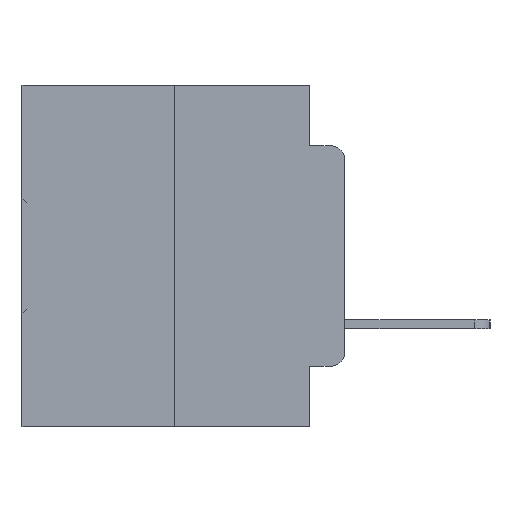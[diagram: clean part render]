
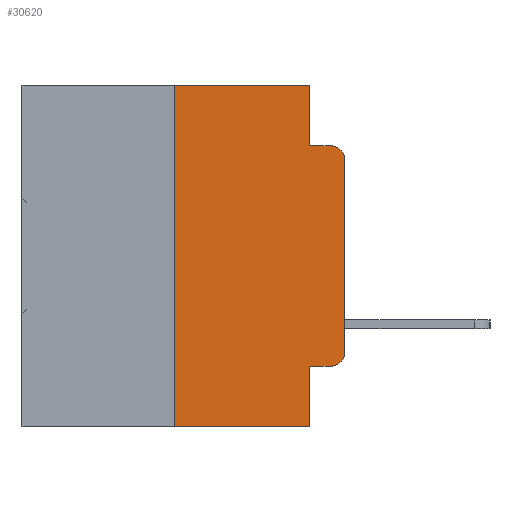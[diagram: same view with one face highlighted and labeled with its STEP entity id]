
A CAD part, left-side view. The second image highlights one B-rep face of the part: STEP entity #30620.
In plain terms, the highlighted planar face has unit normal (-1, 0, 0).
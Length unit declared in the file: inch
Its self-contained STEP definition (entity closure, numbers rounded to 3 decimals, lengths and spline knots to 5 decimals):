
#858 = EDGE_CURVE ( 'NONE', #8218, #5733, #8881, .T. ) ;
#883 = LINE ( 'NONE', #3838, #12982 ) ;
#1168 = EDGE_CURVE ( 'NONE', #4588, #17479, #20511, .T. ) ;
#2217 = DIRECTION ( 'NONE',  ( 0., 0., -1. ) ) ;
#2550 = DIRECTION ( 'NONE',  ( -1., 0., 0. ) ) ;
#2579 = ORIENTED_EDGE ( 'NONE', *, *, #3628, .T. ) ;
#2965 = LINE ( 'NONE', #25758, #28942 ) ;
#3628 = EDGE_CURVE ( 'NONE', #4588, #26644, #7631, .T. ) ;
#3838 = CARTESIAN_POINT ( 'NONE',  ( 0., 0.051, -0.0885 ) ) ;
#4324 = DIRECTION ( 'NONE',  ( 0., 0., 1. ) ) ;
#4588 = VERTEX_POINT ( 'NONE', #18211 ) ;
#5226 = EDGE_CURVE ( 'NONE', #5733, #17076, #21538, .T. ) ;
#5264 = EDGE_CURVE ( 'NONE', #19134, #17076, #883, .T. ) ;
#5346 = DIRECTION ( 'NONE',  ( 0., 0., 1. ) ) ;
#5366 = EDGE_CURVE ( 'NONE', #23782, #19134, #2965, .T. ) ;
#5705 = DIRECTION ( 'NONE',  ( -1., 0., 0. ) ) ;
#5733 = VERTEX_POINT ( 'NONE', #20081 ) ;
#5838 = VECTOR ( 'NONE', #27676, 39.37008 ) ;
#5846 = CARTESIAN_POINT ( 'NONE',  ( 0., 0.473, 0. ) ) ;
#5957 = LINE ( 'NONE', #25473, #25893 ) ;
#6396 = AXIS2_PLACEMENT_3D ( 'NONE', #17402, #5705, #10441 ) ;
#7501 = CARTESIAN_POINT ( 'NONE',  ( 0., 0.051, -0.4115 ) ) ;
#7631 = LINE ( 'NONE', #7501, #32658 ) ;
#7640 = VERTEX_POINT ( 'NONE', #32316 ) ;
#7984 = DIRECTION ( 'NONE',  ( 0., -1., 0. ) ) ;
#8181 = CARTESIAN_POINT ( 'NONE',  ( 0., 0.02, -0.4115 ) ) ;
#8218 = VERTEX_POINT ( 'NONE', #31843 ) ;
#8352 = PLANE ( 'NONE',  #21915 ) ;
#8881 = LINE ( 'NONE', #20272, #22927 ) ;
#9037 = EDGE_CURVE ( 'NONE', #7640, #10175, #15525, .T. ) ;
#9444 = ORIENTED_EDGE ( 'NONE', *, *, #21715, .T. ) ;
#10175 = VERTEX_POINT ( 'NONE', #11527 ) ;
#10441 = DIRECTION ( 'NONE',  ( 0., 0., -1. ) ) ;
#11527 = CARTESIAN_POINT ( 'NONE',  ( 0., 0.25, 0. ) ) ;
#12526 = LINE ( 'NONE', #17604, #5838 ) ;
#12982 = VECTOR ( 'NONE', #28740, 39.37008 ) ;
#13798 = ORIENTED_EDGE ( 'NONE', *, *, #9037, .F. ) ;
#15057 = CARTESIAN_POINT ( 'NONE',  ( 0., 0.051, 0. ) ) ;
#15525 = LINE ( 'NONE', #19328, #24042 ) ;
#15958 = CARTESIAN_POINT ( 'NONE',  ( 0., 0.051, -0.0885 ) ) ;
#17076 = VERTEX_POINT ( 'NONE', #27655 ) ;
#17402 = CARTESIAN_POINT ( 'NONE',  ( 0., 0.02, -0.1085 ) ) ;
#17479 = VERTEX_POINT ( 'NONE', #31328 ) ;
#17604 = CARTESIAN_POINT ( 'NONE',  ( 0., 0.473, -0.5 ) ) ;
#17721 = CARTESIAN_POINT ( 'NONE',  ( 0., 0.02, -0.3915 ) ) ;
#18211 = CARTESIAN_POINT ( 'NONE',  ( 0., 0.051, -0.4115 ) ) ;
#18778 = ORIENTED_EDGE ( 'NONE', *, *, #5366, .F. ) ;
#19088 = CIRCLE ( 'NONE', #28227, 0.02 ) ;
#19134 = VERTEX_POINT ( 'NONE', #15958 ) ;
#19328 = CARTESIAN_POINT ( 'NONE',  ( 0., 0.25, 0. ) ) ;
#19840 = FACE_OUTER_BOUND ( 'NONE', #25358, .T. ) ;
#20081 = CARTESIAN_POINT ( 'NONE',  ( 0., 0., -0.1085 ) ) ;
#20176 = DIRECTION ( 'NONE',  ( 0., 0., -1. ) ) ;
#20272 = CARTESIAN_POINT ( 'NONE',  ( 0., 0., 0. ) ) ;
#20511 = LINE ( 'NONE', #15057, #26450 ) ;
#20934 = CARTESIAN_POINT ( 'NONE',  ( 0., 0.051, 0. ) ) ;
#21538 = CIRCLE ( 'NONE', #6396, 0.02 ) ;
#21711 = EDGE_CURVE ( 'NONE', #7640, #17479, #12526, .T. ) ;
#21715 = EDGE_CURVE ( 'NONE', #26644, #8218, #19088, .T. ) ;
#21895 = ORIENTED_EDGE ( 'NONE', *, *, #1168, .F. ) ;
#21915 = AXIS2_PLACEMENT_3D ( 'NONE', #5846, #23184, #25831 ) ;
#22913 = DIRECTION ( 'NONE',  ( 0., 0., -1. ) ) ;
#22927 = VECTOR ( 'NONE', #5346, 39.37008 ) ;
#23184 = DIRECTION ( 'NONE',  ( 1., 0., 0. ) ) ;
#23782 = VERTEX_POINT ( 'NONE', #20934 ) ;
#23864 = ORIENTED_EDGE ( 'NONE', *, *, #5226, .T. ) ;
#24042 = VECTOR ( 'NONE', #4324, 39.37008 ) ;
#24340 = EDGE_CURVE ( 'NONE', #10175, #23782, #5957, .T. ) ;
#25358 = EDGE_LOOP ( 'NONE', ( #28180, #23864, #30517, #18778, #32089, #13798, #27041, #21895, #2579, #9444 ) ) ;
#25473 = CARTESIAN_POINT ( 'NONE',  ( 0., 0.473, 0. ) ) ;
#25758 = CARTESIAN_POINT ( 'NONE',  ( 0., 0.051, 0. ) ) ;
#25831 = DIRECTION ( 'NONE',  ( 0., 0., -1. ) ) ;
#25893 = VECTOR ( 'NONE', #7984, 39.37008 ) ;
#26450 = VECTOR ( 'NONE', #22913, 39.37008 ) ;
#26644 = VERTEX_POINT ( 'NONE', #8181 ) ;
#27041 = ORIENTED_EDGE ( 'NONE', *, *, #21711, .T. ) ;
#27655 = CARTESIAN_POINT ( 'NONE',  ( 0., 0.02, -0.0885 ) ) ;
#27676 = DIRECTION ( 'NONE',  ( 0., -1., 0. ) ) ;
#28180 = ORIENTED_EDGE ( 'NONE', *, *, #858, .T. ) ;
#28227 = AXIS2_PLACEMENT_3D ( 'NONE', #17721, #2550, #20176 ) ;
#28740 = DIRECTION ( 'NONE',  ( 0., -1., 0. ) ) ;
#28942 = VECTOR ( 'NONE', #2217, 39.37008 ) ;
#30517 = ORIENTED_EDGE ( 'NONE', *, *, #5264, .F. ) ;
#30598 = DIRECTION ( 'NONE',  ( 0., -1., 0. ) ) ;
#30620 = ADVANCED_FACE ( 'NONE', ( #19840 ), #8352, .F. ) ;
#31328 = CARTESIAN_POINT ( 'NONE',  ( 0., 0.051, -0.5 ) ) ;
#31843 = CARTESIAN_POINT ( 'NONE',  ( 0., 0., -0.3915 ) ) ;
#32089 = ORIENTED_EDGE ( 'NONE', *, *, #24340, .F. ) ;
#32316 = CARTESIAN_POINT ( 'NONE',  ( 0., 0.25, -0.5 ) ) ;
#32658 = VECTOR ( 'NONE', #30598, 39.37008 ) ;
